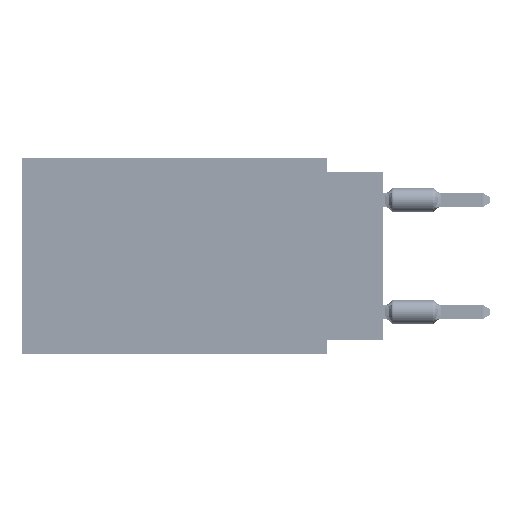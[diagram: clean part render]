
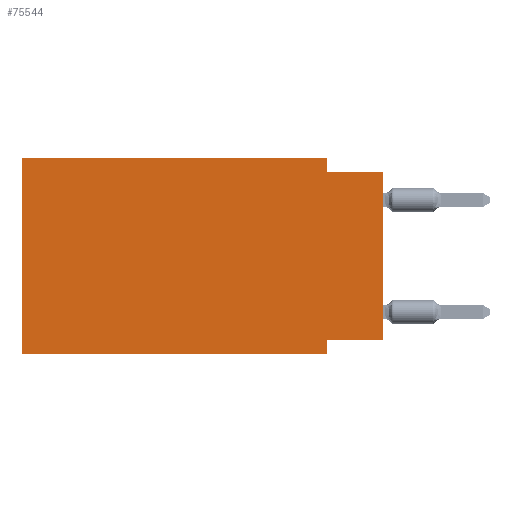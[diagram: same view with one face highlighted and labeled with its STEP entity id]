
A CAD part, left-side view. The second image highlights one B-rep face of the part: STEP entity #75544.
In plain terms, the highlighted planar face has unit normal (-1, 0, 0).
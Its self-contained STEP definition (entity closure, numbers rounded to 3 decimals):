
#332 = EDGE_CURVE ( 'NONE', #23939, #55629, #61155, .T. ) ;
#2033 = FACE_OUTER_BOUND ( 'NONE', #10107, .T. ) ;
#2728 = VERTEX_POINT ( 'NONE', #3798 ) ;
#2923 = VERTEX_POINT ( 'NONE', #76662 ) ;
#3798 = CARTESIAN_POINT ( 'NONE',  ( 0., 2.54, -0.635 ) ) ;
#5418 = DIRECTION ( 'NONE',  ( 0., 0., -1. ) ) ;
#5446 = CARTESIAN_POINT ( 'NONE',  ( 0., 0., 0. ) ) ;
#8064 = ORIENTED_EDGE ( 'NONE', *, *, #74589, .T. ) ;
#8382 = DIRECTION ( 'NONE',  ( 0., 0., -1. ) ) ;
#10107 = EDGE_LOOP ( 'NONE', ( #8064, #44935, #22385, #21137, #33584, #70548, #68420, #14550 ) ) ;
#10257 = CARTESIAN_POINT ( 'NONE',  ( 0., 16.383, -8.89 ) ) ;
#10349 = VECTOR ( 'NONE', #48491, 1000. ) ;
#11112 = AXIS2_PLACEMENT_3D ( 'NONE', #68312, #20320, #8382 ) ;
#12623 = DIRECTION ( 'NONE',  ( 0., 0., -1. ) ) ;
#12943 = CARTESIAN_POINT ( 'NONE',  ( 0., 0., -0.635 ) ) ;
#14550 = ORIENTED_EDGE ( 'NONE', *, *, #332, .F. ) ;
#14612 = VECTOR ( 'NONE', #49482, 1000. ) ;
#15446 = LINE ( 'NONE', #10257, #68973 ) ;
#15797 = CARTESIAN_POINT ( 'NONE',  ( 0., 0., -0.635 ) ) ;
#19095 = CARTESIAN_POINT ( 'NONE',  ( 0., 0., -8.255 ) ) ;
#19949 = CARTESIAN_POINT ( 'NONE',  ( 0., 16.383, 0. ) ) ;
#20320 = DIRECTION ( 'NONE',  ( 1., 0., 0. ) ) ;
#21137 = ORIENTED_EDGE ( 'NONE', *, *, #55296, .F. ) ;
#21198 = VERTEX_POINT ( 'NONE', #32768 ) ;
#22385 = ORIENTED_EDGE ( 'NONE', *, *, #33315, .F. ) ;
#23939 = VERTEX_POINT ( 'NONE', #59687 ) ;
#24556 = CARTESIAN_POINT ( 'NONE',  ( 0., 2.54, -8.89 ) ) ;
#25111 = DIRECTION ( 'NONE',  ( 0., 0., 1. ) ) ;
#25268 = LINE ( 'NONE', #12943, #14612 ) ;
#26262 = PLANE ( 'NONE',  #11112 ) ;
#26591 = CARTESIAN_POINT ( 'NONE',  ( 0., 2.54, 0. ) ) ;
#28130 = VERTEX_POINT ( 'NONE', #72928 ) ;
#28778 = VECTOR ( 'NONE', #66896, 1000. ) ;
#29744 = LINE ( 'NONE', #24556, #64293 ) ;
#30800 = LINE ( 'NONE', #41933, #75719 ) ;
#31168 = CARTESIAN_POINT ( 'NONE',  ( 0., 16.383, 0. ) ) ;
#32768 = CARTESIAN_POINT ( 'NONE',  ( 0., 16.383, 0. ) ) ;
#32841 = EDGE_CURVE ( 'NONE', #55629, #28130, #29744, .T. ) ;
#33315 = EDGE_CURVE ( 'NONE', #38751, #2728, #30800, .T. ) ;
#33584 = ORIENTED_EDGE ( 'NONE', *, *, #43922, .F. ) ;
#38751 = VERTEX_POINT ( 'NONE', #26591 ) ;
#41440 = CARTESIAN_POINT ( 'NONE',  ( 0., 2.54, -8.255 ) ) ;
#41933 = CARTESIAN_POINT ( 'NONE',  ( 0., 2.54, 0. ) ) ;
#43922 = EDGE_CURVE ( 'NONE', #2923, #21198, #61206, .T. ) ;
#44935 = ORIENTED_EDGE ( 'NONE', *, *, #51569, .F. ) ;
#45241 = VECTOR ( 'NONE', #55030, 1000. ) ;
#47630 = VERTEX_POINT ( 'NONE', #15797 ) ;
#48491 = DIRECTION ( 'NONE',  ( 0., 1., 0. ) ) ;
#49482 = DIRECTION ( 'NONE',  ( 0., -1., 0. ) ) ;
#50113 = EDGE_CURVE ( 'NONE', #2923, #28130, #15446, .T. ) ;
#51569 = EDGE_CURVE ( 'NONE', #2728, #47630, #25268, .T. ) ;
#51583 = DIRECTION ( 'NONE',  ( 0., -1., 0. ) ) ;
#52020 = VECTOR ( 'NONE', #25111, 1000. ) ;
#55030 = DIRECTION ( 'NONE',  ( 0., 0., 1. ) ) ;
#55296 = EDGE_CURVE ( 'NONE', #21198, #38751, #66128, .T. ) ;
#55629 = VERTEX_POINT ( 'NONE', #41440 ) ;
#59687 = CARTESIAN_POINT ( 'NONE',  ( 0., 0., -8.255 ) ) ;
#61155 = LINE ( 'NONE', #19095, #10349 ) ;
#61206 = LINE ( 'NONE', #19949, #52020 ) ;
#64293 = VECTOR ( 'NONE', #12623, 1000. ) ;
#66128 = LINE ( 'NONE', #31168, #28778 ) ;
#66896 = DIRECTION ( 'NONE',  ( 0., -1., 0. ) ) ;
#67312 = LINE ( 'NONE', #5446, #45241 ) ;
#68312 = CARTESIAN_POINT ( 'NONE',  ( 0., 16.383, 0. ) ) ;
#68420 = ORIENTED_EDGE ( 'NONE', *, *, #32841, .F. ) ;
#68973 = VECTOR ( 'NONE', #51583, 1000. ) ;
#70548 = ORIENTED_EDGE ( 'NONE', *, *, #50113, .T. ) ;
#72928 = CARTESIAN_POINT ( 'NONE',  ( 0., 2.54, -8.89 ) ) ;
#74589 = EDGE_CURVE ( 'NONE', #23939, #47630, #67312, .T. ) ;
#75544 = ADVANCED_FACE ( 'NONE', ( #2033 ), #26262, .F. ) ;
#75719 = VECTOR ( 'NONE', #5418, 1000. ) ;
#76662 = CARTESIAN_POINT ( 'NONE',  ( 0., 16.383, -8.89 ) ) ;
